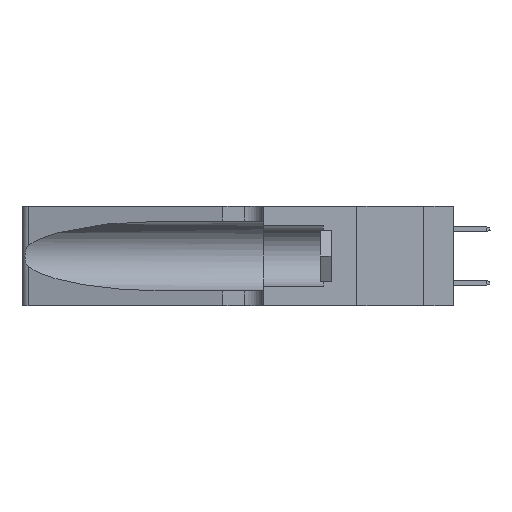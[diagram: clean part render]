
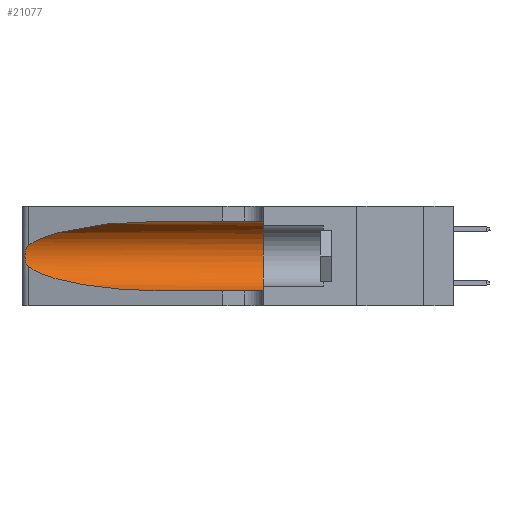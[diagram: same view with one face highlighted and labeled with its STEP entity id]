
A CAD part, left-side view. The second image highlights one B-rep face of the part: STEP entity #21077.
In plain terms, the highlighted cylindrical face has radius 3.308 mm (diameter 6.617 mm), a partial arc.
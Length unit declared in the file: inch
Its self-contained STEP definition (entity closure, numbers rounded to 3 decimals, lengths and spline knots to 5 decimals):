
#380 = CARTESIAN_POINT ( 'NONE',  ( 0.25487, 1.22718, 0.14631 ) ) ;
#439 = CARTESIAN_POINT ( 'NONE',  ( 0.25487, 1.22718, 0.22369 ) ) ;
#875 = VERTEX_POINT ( 'NONE', #28975 ) ;
#1030 = DIRECTION ( 'NONE',  ( 0., -1., 0. ) ) ;
#1224 = CARTESIAN_POINT ( 'NONE',  ( 0.1305, 0.72297, 0.05475 ) ) ;
#2141 = DIRECTION ( 'NONE',  ( 0., -1., 0. ) ) ;
#2285 = ORIENTED_EDGE ( 'NONE', *, *, #8876, .T. ) ;
#2811 = CARTESIAN_POINT ( 'NONE',  ( 0.25639, 1.23186, 0.15144 ) ) ;
#3311 = CIRCLE ( 'NONE', #28363, 0.13025 ) ;
#3714 = EDGE_CURVE ( 'NONE', #19938, #34097, #13265, .T. ) ;
#5363 = CARTESIAN_POINT ( 'NONE',  ( 0.26075, 1.23896, 0.178 ) ) ;
#5538 = CARTESIAN_POINT ( 'NONE',  ( 0.25854, 1.2359, 0.20912 ) ) ;
#6608 = DIRECTION ( 'NONE',  ( 0., -1., 0. ) ) ;
#6783 = CARTESIAN_POINT ( 'NONE',  ( 0.1305, 1.61858, 0.185 ) ) ;
#7632 =( BOUNDED_CURVE ( )  B_SPLINE_CURVE ( 3, ( #15697, #12408, #20793, #34619 ),
 .UNSPECIFIED., .F., .T. ) 
 B_SPLINE_CURVE_WITH_KNOTS ( ( 4, 4 ),
 ( 1.5708, 2.84003 ),
 .UNSPECIFIED. ) 
 CURVE ( )  GEOMETRIC_REPRESENTATION_ITEM ( )  RATIONAL_B_SPLINE_CURVE ( ( 1., 0.87, 0.87, 1. ) ) 
 REPRESENTATION_ITEM ( '' )  );
#7828 = VECTOR ( 'NONE', #1030, 39.37008 ) ;
#8109 = CARTESIAN_POINT ( 'NONE',  ( 0.25787, 1.23484, 0.2124 ) ) ;
#8876 = EDGE_CURVE ( 'NONE', #11956, #35879, #33703, .T. ) ;
#8973 = CARTESIAN_POINT ( 'NONE',  ( 0.1305, 0.72297, 0.05475 ) ) ;
#10840 = CARTESIAN_POINT ( 'NONE',  ( 0.25639, 1.23184, 0.21858 ) ) ;
#11116 = CARTESIAN_POINT ( 'NONE',  ( 0.25487, 1.22718, 0.14631 ) ) ;
#11216 = CARTESIAN_POINT ( 'NONE',  ( 0.1305, 0.35, 0.31525 ) ) ;
#11508 = CARTESIAN_POINT ( 'NONE',  ( 0.2373, 1.15595, 0.08982 ) ) ;
#11883 = FACE_OUTER_BOUND ( 'NONE', #35113, .T. ) ;
#11956 = VERTEX_POINT ( 'NONE', #11116 ) ;
#12387 = CARTESIAN_POINT ( 'NONE',  ( 0.1305, 0.35, 0.185 ) ) ;
#12408 = CARTESIAN_POINT ( 'NONE',  ( 0.18966, 0.96281, 0.31525 ) ) ;
#13265 = LINE ( 'NONE', #19269, #14060 ) ;
#13461 = EDGE_CURVE ( 'NONE', #34097, #875, #3311, .T. ) ;
#13938 = CARTESIAN_POINT ( 'NONE',  ( 0.25555, 1.22993, 0.14849 ) ) ;
#14060 = VECTOR ( 'NONE', #2141, 39.37008 ) ;
#15319 = DIRECTION ( 'NONE',  ( 0., 0., 1. ) ) ;
#15697 = CARTESIAN_POINT ( 'NONE',  ( 0.1305, 0.72297, 0.31525 ) ) ;
#16499 = CARTESIAN_POINT ( 'NONE',  ( 0.25789, 1.23486, 0.15765 ) ) ;
#16621 = CARTESIAN_POINT ( 'NONE',  ( 0.18966, 0.96281, 0.05475 ) ) ;
#16676 = CARTESIAN_POINT ( 'NONE',  ( 0.26017, 1.23833, 0.17102 ) ) ;
#18843 = EDGE_CURVE ( 'NONE', #35879, #875, #34015, .T. ) ;
#18989 = ORIENTED_EDGE ( 'NONE', *, *, #33493, .T. ) ;
#19229 = CARTESIAN_POINT ( 'NONE',  ( 0.26018, 1.23835, 0.19895 ) ) ;
#19269 = CARTESIAN_POINT ( 'NONE',  ( 0.1305, 1.61858, 0.31525 ) ) ;
#19938 = VERTEX_POINT ( 'NONE', #29575 ) ;
#19946 = ORIENTED_EDGE ( 'NONE', *, *, #18843, .T. ) ;
#19959 = B_SPLINE_CURVE_WITH_KNOTS ( 'NONE', 3,
 ( #439, #27449, #10840, #8109, #5538, #19229, #30356, #5363, #16676, #27811, #16499, #2811, #13938, #25069 ),
 .UNSPECIFIED., .F., .F.,
 ( 4, 2, 2, 2, 2, 2, 4 ),
 ( 0., 0.00027, 0.00053, 0.00107, 0.0016, 0.00187, 0.00214 ),
 .UNSPECIFIED. ) ;
#20633 = CYLINDRICAL_SURFACE ( 'NONE', #23666, 0.13025 ) ;
#20793 = CARTESIAN_POINT ( 'NONE',  ( 0.2373, 1.15595, 0.28018 ) ) ;
#21077 = ADVANCED_FACE ( 'NONE', ( #11883 ), #20633, .F. ) ;
#22440 = ORIENTED_EDGE ( 'NONE', *, *, #3714, .F. ) ;
#23666 = AXIS2_PLACEMENT_3D ( 'NONE', #6783, #6608, #31583 ) ;
#24108 = VERTEX_POINT ( 'NONE', #27213 ) ;
#25069 = CARTESIAN_POINT ( 'NONE',  ( 0.25487, 1.22718, 0.14631 ) ) ;
#26036 = CARTESIAN_POINT ( 'NONE',  ( 0.1305, 1.61858, 0.05475 ) ) ;
#27213 = CARTESIAN_POINT ( 'NONE',  ( 0.25487, 1.22718, 0.22369 ) ) ;
#27449 = CARTESIAN_POINT ( 'NONE',  ( 0.25555, 1.22994, 0.2215 ) ) ;
#27498 = ORIENTED_EDGE ( 'NONE', *, *, #13461, .F. ) ;
#27811 = CARTESIAN_POINT ( 'NONE',  ( 0.25856, 1.23593, 0.16098 ) ) ;
#28234 = ORIENTED_EDGE ( 'NONE', *, *, #29740, .T. ) ;
#28363 = AXIS2_PLACEMENT_3D ( 'NONE', #12387, #34958, #15319 ) ;
#28975 = CARTESIAN_POINT ( 'NONE',  ( 0.1305, 0.35, 0.05475 ) ) ;
#29575 = CARTESIAN_POINT ( 'NONE',  ( 0.1305, 0.72297, 0.31525 ) ) ;
#29740 = EDGE_CURVE ( 'NONE', #24108, #11956, #19959, .T. ) ;
#30356 = CARTESIAN_POINT ( 'NONE',  ( 0.26075, 1.23896, 0.19203 ) ) ;
#31583 = DIRECTION ( 'NONE',  ( 0., 0., -1. ) ) ;
#33493 = EDGE_CURVE ( 'NONE', #19938, #24108, #7632, .T. ) ;
#33703 =( BOUNDED_CURVE ( )  B_SPLINE_CURVE ( 3, ( #380, #11508, #16621, #8973 ),
 .UNSPECIFIED., .F., .T. ) 
 B_SPLINE_CURVE_WITH_KNOTS ( ( 4, 4 ),
 ( 3.44316, 4.71239 ),
 .UNSPECIFIED. ) 
 CURVE ( )  GEOMETRIC_REPRESENTATION_ITEM ( )  RATIONAL_B_SPLINE_CURVE ( ( 1., 0.87, 0.87, 1. ) ) 
 REPRESENTATION_ITEM ( '' )  );
#34015 = LINE ( 'NONE', #26036, #7828 ) ;
#34097 = VERTEX_POINT ( 'NONE', #11216 ) ;
#34619 = CARTESIAN_POINT ( 'NONE',  ( 0.25487, 1.22718, 0.22369 ) ) ;
#34958 = DIRECTION ( 'NONE',  ( 0., 1., 0. ) ) ;
#35113 = EDGE_LOOP ( 'NONE', ( #18989, #28234, #2285, #19946, #27498, #22440 ) ) ;
#35879 = VERTEX_POINT ( 'NONE', #1224 ) ;
